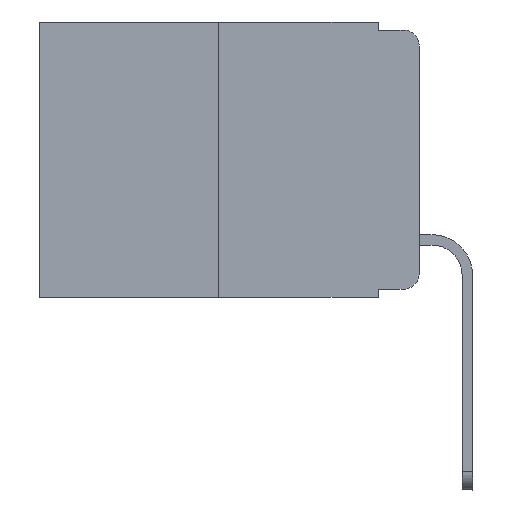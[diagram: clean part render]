
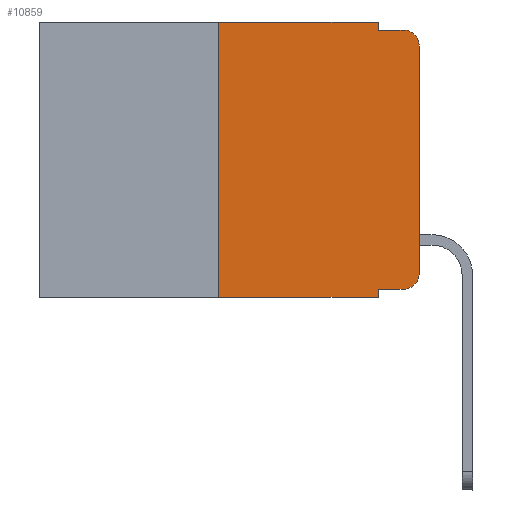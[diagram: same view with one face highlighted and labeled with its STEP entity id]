
A CAD part, left-side view. The second image highlights one B-rep face of the part: STEP entity #10859.
In plain terms, the highlighted planar face has unit normal (-1, 0, 0).
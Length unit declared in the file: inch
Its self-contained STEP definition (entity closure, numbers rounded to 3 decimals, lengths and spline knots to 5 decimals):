
#125 = EDGE_CURVE ( 'NONE', #6979, #3499, #2935, .T. ) ;
#147 = DIRECTION ( 'NONE',  ( 0., 0., -1. ) ) ;
#209 = CARTESIAN_POINT ( 'NONE',  ( 0., 0.051, -0.333 ) ) ;
#261 = DIRECTION ( 'NONE',  ( 0., -1., 0. ) ) ;
#431 = DIRECTION ( 'NONE',  ( 0., 0., -1. ) ) ;
#563 = LINE ( 'NONE', #14140, #2203 ) ;
#593 = VECTOR ( 'NONE', #2779, 39.37008 ) ;
#772 = PLANE ( 'NONE',  #9568 ) ;
#846 = DIRECTION ( 'NONE',  ( 0., 0., -1. ) ) ;
#1457 = EDGE_CURVE ( 'NONE', #5320, #6851, #14266, .T. ) ;
#1730 = EDGE_CURVE ( 'NONE', #7619, #11852, #10651, .T. ) ;
#1863 = EDGE_CURVE ( 'NONE', #5028, #6979, #5412, .T. ) ;
#1902 = EDGE_CURVE ( 'NONE', #11572, #12919, #11105, .T. ) ;
#2129 = CARTESIAN_POINT ( 'NONE',  ( 0., 0., -0.313 ) ) ;
#2203 = VECTOR ( 'NONE', #261, 39.37008 ) ;
#2453 = VECTOR ( 'NONE', #147, 39.37008 ) ;
#2779 = DIRECTION ( 'NONE',  ( 0., -1., 0. ) ) ;
#2839 = EDGE_CURVE ( 'NONE', #5028, #11852, #8254, .T. ) ;
#2935 = LINE ( 'NONE', #9841, #593 ) ;
#2992 = DIRECTION ( 'NONE',  ( 0., -1., 0. ) ) ;
#3351 = VECTOR ( 'NONE', #7045, 39.37008 ) ;
#3362 = LINE ( 'NONE', #11393, #3351 ) ;
#3499 = VERTEX_POINT ( 'NONE', #4171 ) ;
#3857 = CARTESIAN_POINT ( 'NONE',  ( 0., 0.25, -0.343 ) ) ;
#3973 = DIRECTION ( 'NONE',  ( 0., 0., -1. ) ) ;
#3980 = CARTESIAN_POINT ( 'NONE',  ( 0., 0., 0. ) ) ;
#4042 = AXIS2_PLACEMENT_3D ( 'NONE', #14258, #7221, #3973 ) ;
#4063 = CARTESIAN_POINT ( 'NONE',  ( 0., 0.25, 0. ) ) ;
#4171 = CARTESIAN_POINT ( 'NONE',  ( 0., 0.051, 0. ) ) ;
#4210 = FACE_OUTER_BOUND ( 'NONE', #8008, .T. ) ;
#4287 = DIRECTION ( 'NONE',  ( 1., 0., 0. ) ) ;
#4705 = EDGE_CURVE ( 'NONE', #6824, #5320, #13603, .T. ) ;
#5028 = VERTEX_POINT ( 'NONE', #3857 ) ;
#5320 = VERTEX_POINT ( 'NONE', #2129 ) ;
#5412 = LINE ( 'NONE', #11022, #13476 ) ;
#5511 = ORIENTED_EDGE ( 'NONE', *, *, #1863, .F. ) ;
#5537 = ORIENTED_EDGE ( 'NONE', *, *, #10329, .T. ) ;
#5593 = VECTOR ( 'NONE', #8568, 39.37008 ) ;
#5948 = AXIS2_PLACEMENT_3D ( 'NONE', #6146, #7190, #431 ) ;
#6146 = CARTESIAN_POINT ( 'NONE',  ( 0., 0.02, -0.313 ) ) ;
#6824 = VERTEX_POINT ( 'NONE', #11878 ) ;
#6843 = DIRECTION ( 'NONE',  ( 0., -1., 0. ) ) ;
#6851 = VERTEX_POINT ( 'NONE', #7531 ) ;
#6979 = VERTEX_POINT ( 'NONE', #4063 ) ;
#7045 = DIRECTION ( 'NONE',  ( 0., 0., -1. ) ) ;
#7136 = CARTESIAN_POINT ( 'NONE',  ( 0., 0.051, 0. ) ) ;
#7190 = DIRECTION ( 'NONE',  ( -1., 0., 0. ) ) ;
#7221 = DIRECTION ( 'NONE',  ( -1., 0., 0. ) ) ;
#7531 = CARTESIAN_POINT ( 'NONE',  ( 0., 0., -0.03 ) ) ;
#7619 = VERTEX_POINT ( 'NONE', #209 ) ;
#8008 = EDGE_LOOP ( 'NONE', ( #14499, #5537, #9996, #10229, #10400, #5511, #11814, #9651, #10643, #11128 ) ) ;
#8254 = LINE ( 'NONE', #13733, #13987 ) ;
#8387 = CARTESIAN_POINT ( 'NONE',  ( 0., 0.051, -0.01 ) ) ;
#8568 = DIRECTION ( 'NONE',  ( 0., 0., 1. ) ) ;
#9088 = CIRCLE ( 'NONE', #4042, 0.02 ) ;
#9568 = AXIS2_PLACEMENT_3D ( 'NONE', #11118, #4287, #846 ) ;
#9651 = ORIENTED_EDGE ( 'NONE', *, *, #1730, .F. ) ;
#9841 = CARTESIAN_POINT ( 'NONE',  ( 0., 0.473, 0. ) ) ;
#9996 = ORIENTED_EDGE ( 'NONE', *, *, #1902, .F. ) ;
#10229 = ORIENTED_EDGE ( 'NONE', *, *, #11434, .F. ) ;
#10329 = EDGE_CURVE ( 'NONE', #6851, #12919, #9088, .T. ) ;
#10400 = ORIENTED_EDGE ( 'NONE', *, *, #125, .F. ) ;
#10643 = ORIENTED_EDGE ( 'NONE', *, *, #13155, .T. ) ;
#10651 = LINE ( 'NONE', #7136, #2453 ) ;
#10859 = ADVANCED_FACE ( 'NONE', ( #4210 ), #772, .F. ) ;
#11022 = CARTESIAN_POINT ( 'NONE',  ( 0., 0.25, 0. ) ) ;
#11105 = LINE ( 'NONE', #13277, #13691 ) ;
#11118 = CARTESIAN_POINT ( 'NONE',  ( 0., 0.473, 0. ) ) ;
#11128 = ORIENTED_EDGE ( 'NONE', *, *, #4705, .T. ) ;
#11393 = CARTESIAN_POINT ( 'NONE',  ( 0., 0.051, 0. ) ) ;
#11434 = EDGE_CURVE ( 'NONE', #3499, #11572, #3362, .T. ) ;
#11572 = VERTEX_POINT ( 'NONE', #8387 ) ;
#11814 = ORIENTED_EDGE ( 'NONE', *, *, #2839, .T. ) ;
#11852 = VERTEX_POINT ( 'NONE', #12573 ) ;
#11878 = CARTESIAN_POINT ( 'NONE',  ( 0., 0.02, -0.333 ) ) ;
#12428 = CARTESIAN_POINT ( 'NONE',  ( 0., 0.02, -0.01 ) ) ;
#12573 = CARTESIAN_POINT ( 'NONE',  ( 0., 0.051, -0.343 ) ) ;
#12919 = VERTEX_POINT ( 'NONE', #12428 ) ;
#13155 = EDGE_CURVE ( 'NONE', #7619, #6824, #563, .T. ) ;
#13277 = CARTESIAN_POINT ( 'NONE',  ( 0., 0.051, -0.01 ) ) ;
#13476 = VECTOR ( 'NONE', #14252, 39.37008 ) ;
#13603 = CIRCLE ( 'NONE', #5948, 0.02 ) ;
#13691 = VECTOR ( 'NONE', #2992, 39.37008 ) ;
#13733 = CARTESIAN_POINT ( 'NONE',  ( 0., 0.473, -0.343 ) ) ;
#13987 = VECTOR ( 'NONE', #6843, 39.37008 ) ;
#14140 = CARTESIAN_POINT ( 'NONE',  ( 0., 0.051, -0.333 ) ) ;
#14252 = DIRECTION ( 'NONE',  ( 0., 0., 1. ) ) ;
#14258 = CARTESIAN_POINT ( 'NONE',  ( 0., 0.02, -0.03 ) ) ;
#14266 = LINE ( 'NONE', #3980, #5593 ) ;
#14499 = ORIENTED_EDGE ( 'NONE', *, *, #1457, .T. ) ;
